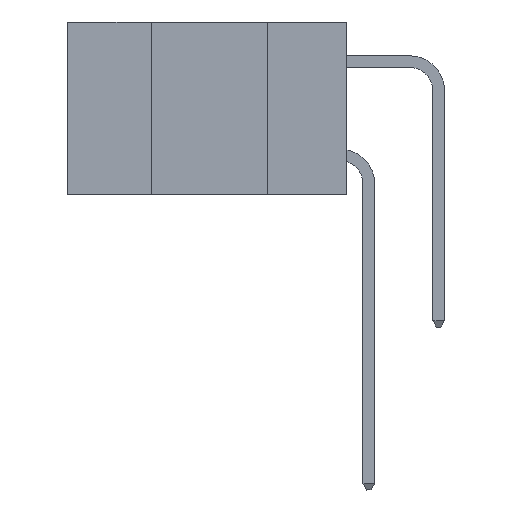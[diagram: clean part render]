
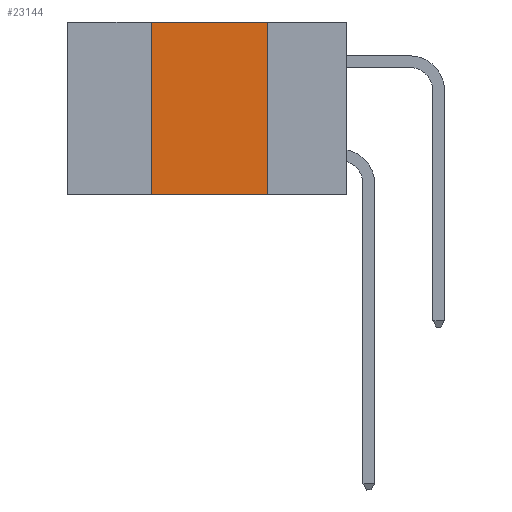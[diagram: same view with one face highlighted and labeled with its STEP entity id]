
A CAD part, left-side view. The second image highlights one B-rep face of the part: STEP entity #23144.
In plain terms, the highlighted planar face has unit normal (-1, 0, 0).
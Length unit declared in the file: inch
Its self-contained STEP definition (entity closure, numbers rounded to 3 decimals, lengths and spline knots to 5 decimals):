
#994 = DIRECTION ( 'NONE',  ( 1., 0., 0. ) ) ;
#1447 = DIRECTION ( 'NONE',  ( 0., 0., 1. ) ) ;
#1515 = DIRECTION ( 'NONE',  ( 0., -1., 0. ) ) ;
#2189 = CARTESIAN_POINT ( 'NONE',  ( 0., 0.6, -0.37 ) ) ;
#3776 = CARTESIAN_POINT ( 'NONE',  ( 0., 0.17, 0. ) ) ;
#4419 = CARTESIAN_POINT ( 'NONE',  ( 0., 0.17, 0. ) ) ;
#4620 = CARTESIAN_POINT ( 'NONE',  ( 0., 0.42, 0. ) ) ;
#4784 = DIRECTION ( 'NONE',  ( 0., 0., -1. ) ) ;
#4868 = CARTESIAN_POINT ( 'NONE',  ( 0., 0.6, 0. ) ) ;
#5845 = ORIENTED_EDGE ( 'NONE', *, *, #19218, .T. ) ;
#6383 = EDGE_CURVE ( 'NONE', #14908, #19418, #11671, .T. ) ;
#6490 = CARTESIAN_POINT ( 'NONE',  ( 0., 0.42, 0. ) ) ;
#7108 = LINE ( 'NONE', #16064, #16566 ) ;
#7381 = VECTOR ( 'NONE', #1447, 39.37008 ) ;
#7597 = EDGE_CURVE ( 'NONE', #20631, #9700, #12470, .T. ) ;
#7668 = DIRECTION ( 'NONE',  ( 0., 0., -1. ) ) ;
#8077 = AXIS2_PLACEMENT_3D ( 'NONE', #4868, #994, #4784 ) ;
#9700 = VERTEX_POINT ( 'NONE', #11853 ) ;
#10631 = ORIENTED_EDGE ( 'NONE', *, *, #7597, .F. ) ;
#11671 = LINE ( 'NONE', #6490, #7381 ) ;
#11853 = CARTESIAN_POINT ( 'NONE',  ( 0., 0.17, -0.37 ) ) ;
#12470 = LINE ( 'NONE', #3776, #22707 ) ;
#14291 = CARTESIAN_POINT ( 'NONE',  ( 0., 0.42, -0.37 ) ) ;
#14908 = VERTEX_POINT ( 'NONE', #14291 ) ;
#15852 = FACE_OUTER_BOUND ( 'NONE', #18017, .T. ) ;
#16064 = CARTESIAN_POINT ( 'NONE',  ( 0., 0.6, 0. ) ) ;
#16097 = EDGE_CURVE ( 'NONE', #19418, #20631, #7108, .T. ) ;
#16566 = VECTOR ( 'NONE', #1515, 39.37008 ) ;
#16976 = ORIENTED_EDGE ( 'NONE', *, *, #16097, .F. ) ;
#18017 = EDGE_LOOP ( 'NONE', ( #10631, #16976, #18574, #5845 ) ) ;
#18268 = VECTOR ( 'NONE', #18490, 39.37008 ) ;
#18490 = DIRECTION ( 'NONE',  ( 0., -1., 0. ) ) ;
#18574 = ORIENTED_EDGE ( 'NONE', *, *, #6383, .F. ) ;
#19218 = EDGE_CURVE ( 'NONE', #14908, #9700, #21731, .T. ) ;
#19418 = VERTEX_POINT ( 'NONE', #4620 ) ;
#19423 = PLANE ( 'NONE',  #8077 ) ;
#20631 = VERTEX_POINT ( 'NONE', #4419 ) ;
#21731 = LINE ( 'NONE', #2189, #18268 ) ;
#22707 = VECTOR ( 'NONE', #7668, 39.37008 ) ;
#23144 = ADVANCED_FACE ( 'NONE', ( #15852 ), #19423, .F. ) ;
